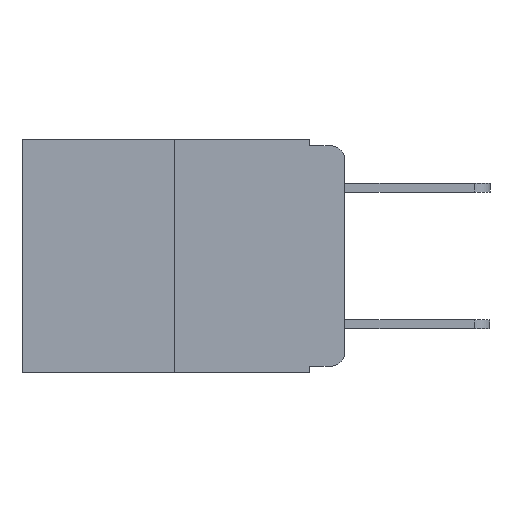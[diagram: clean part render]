
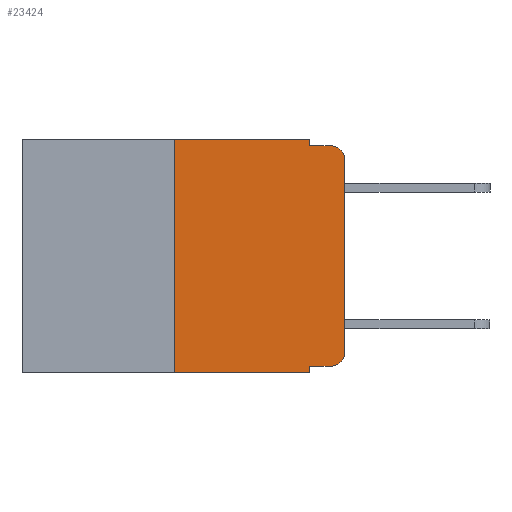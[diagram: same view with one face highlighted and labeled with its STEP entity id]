
A CAD part, left-side view. The second image highlights one B-rep face of the part: STEP entity #23424.
In plain terms, the highlighted planar face has unit normal (-1, 0, 0).
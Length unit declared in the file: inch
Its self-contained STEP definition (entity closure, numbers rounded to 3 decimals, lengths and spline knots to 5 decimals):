
#419 = ORIENTED_EDGE ( 'NONE', *, *, #24900, .T. ) ;
#865 = CARTESIAN_POINT ( 'NONE',  ( 0., 0.473, 0. ) ) ;
#1643 = EDGE_CURVE ( 'NONE', #17742, #3914, #18968, .T. ) ;
#1925 = DIRECTION ( 'NONE',  ( 0., 0., 1. ) ) ;
#2193 = VERTEX_POINT ( 'NONE', #24155 ) ;
#2943 = DIRECTION ( 'NONE',  ( 0., 0., -1. ) ) ;
#3351 = DIRECTION ( 'NONE',  ( 0., 0., 1. ) ) ;
#3469 = ORIENTED_EDGE ( 'NONE', *, *, #14323, .T. ) ;
#3758 = CARTESIAN_POINT ( 'NONE',  ( 0., 0.473, 0. ) ) ;
#3770 = VECTOR ( 'NONE', #12213, 39.37008 ) ;
#3914 = VERTEX_POINT ( 'NONE', #16038 ) ;
#4097 = VERTEX_POINT ( 'NONE', #6999 ) ;
#4697 = VECTOR ( 'NONE', #1925, 39.37008 ) ;
#5209 = CARTESIAN_POINT ( 'NONE',  ( 0., 0.051, -0.343 ) ) ;
#5333 = LINE ( 'NONE', #25013, #20034 ) ;
#5467 = VERTEX_POINT ( 'NONE', #17161 ) ;
#5901 = DIRECTION ( 'NONE',  ( 0., -1., 0. ) ) ;
#6347 = VECTOR ( 'NONE', #17176, 39.37008 ) ;
#6741 = CARTESIAN_POINT ( 'NONE',  ( 0., 0.02, -0.333 ) ) ;
#6977 = CARTESIAN_POINT ( 'NONE',  ( 0., 0., -0.313 ) ) ;
#6999 = CARTESIAN_POINT ( 'NONE',  ( 0., 0.25, -0.343 ) ) ;
#7034 = CARTESIAN_POINT ( 'NONE',  ( 0., 0.02, -0.03 ) ) ;
#7684 = ORIENTED_EDGE ( 'NONE', *, *, #1643, .T. ) ;
#7804 = CARTESIAN_POINT ( 'NONE',  ( 0., 0.051, -0.333 ) ) ;
#8834 = VECTOR ( 'NONE', #3351, 39.37008 ) ;
#8960 = ORIENTED_EDGE ( 'NONE', *, *, #20356, .F. ) ;
#8981 = DIRECTION ( 'NONE',  ( 0., 0., -1. ) ) ;
#9098 = FACE_OUTER_BOUND ( 'NONE', #17158, .T. ) ;
#9564 = CIRCLE ( 'NONE', #15900, 0.02 ) ;
#9618 = EDGE_CURVE ( 'NONE', #5467, #18698, #13600, .T. ) ;
#9799 = DIRECTION ( 'NONE',  ( 0., 0., -1. ) ) ;
#10622 = CARTESIAN_POINT ( 'NONE',  ( 0., 0.02, -0.313 ) ) ;
#10915 = CARTESIAN_POINT ( 'NONE',  ( 0., 0.051, -0.01 ) ) ;
#11240 = CARTESIAN_POINT ( 'NONE',  ( 0., 0.051, 0. ) ) ;
#11308 = EDGE_CURVE ( 'NONE', #18698, #2193, #14424, .T. ) ;
#11548 = CARTESIAN_POINT ( 'NONE',  ( 0., 0.051, -0.333 ) ) ;
#11971 = LINE ( 'NONE', #3758, #6347 ) ;
#12013 = VERTEX_POINT ( 'NONE', #11548 ) ;
#12213 = DIRECTION ( 'NONE',  ( 0., -1., 0. ) ) ;
#12344 = CARTESIAN_POINT ( 'NONE',  ( 0., 0.25, 0. ) ) ;
#12519 = DIRECTION ( 'NONE',  ( 0., 0., -1. ) ) ;
#12824 = VECTOR ( 'NONE', #5901, 39.37008 ) ;
#12828 = DIRECTION ( 'NONE',  ( 0., -1., 0. ) ) ;
#13600 = LINE ( 'NONE', #11240, #18097 ) ;
#14323 = EDGE_CURVE ( 'NONE', #21221, #17742, #23177, .T. ) ;
#14424 = LINE ( 'NONE', #10915, #24014 ) ;
#14495 = DIRECTION ( 'NONE',  ( 1., 0., 0. ) ) ;
#14873 = CARTESIAN_POINT ( 'NONE',  ( 0., 0., 0. ) ) ;
#15462 = ORIENTED_EDGE ( 'NONE', *, *, #24575, .F. ) ;
#15900 = AXIS2_PLACEMENT_3D ( 'NONE', #7034, #20422, #8981 ) ;
#16038 = CARTESIAN_POINT ( 'NONE',  ( 0., 0., -0.03 ) ) ;
#16316 = ORIENTED_EDGE ( 'NONE', *, *, #17960, .F. ) ;
#16337 = PLANE ( 'NONE',  #19644 ) ;
#17153 = VERTEX_POINT ( 'NONE', #5209 ) ;
#17158 = EDGE_LOOP ( 'NONE', ( #7684, #419, #24109, #19073, #16316, #8960, #22121, #15462, #19146, #3469 ) ) ;
#17161 = CARTESIAN_POINT ( 'NONE',  ( 0., 0.051, 0. ) ) ;
#17176 = DIRECTION ( 'NONE',  ( 0., -1., 0. ) ) ;
#17742 = VERTEX_POINT ( 'NONE', #6977 ) ;
#17888 = LINE ( 'NONE', #21809, #3770 ) ;
#17917 = LINE ( 'NONE', #7804, #12824 ) ;
#17960 = EDGE_CURVE ( 'NONE', #23346, #5467, #11971, .T. ) ;
#18097 = VECTOR ( 'NONE', #20932, 39.37008 ) ;
#18698 = VERTEX_POINT ( 'NONE', #23525 ) ;
#18968 = LINE ( 'NONE', #14873, #8834 ) ;
#19040 = EDGE_CURVE ( 'NONE', #12013, #21221, #17917, .T. ) ;
#19073 = ORIENTED_EDGE ( 'NONE', *, *, #9618, .F. ) ;
#19146 = ORIENTED_EDGE ( 'NONE', *, *, #19040, .T. ) ;
#19194 = AXIS2_PLACEMENT_3D ( 'NONE', #10622, #23966, #12519 ) ;
#19644 = AXIS2_PLACEMENT_3D ( 'NONE', #865, #14495, #2943 ) ;
#19676 = LINE ( 'NONE', #24997, #4697 ) ;
#20034 = VECTOR ( 'NONE', #9799, 39.37008 ) ;
#20356 = EDGE_CURVE ( 'NONE', #4097, #23346, #19676, .T. ) ;
#20422 = DIRECTION ( 'NONE',  ( -1., 0., 0. ) ) ;
#20932 = DIRECTION ( 'NONE',  ( 0., 0., -1. ) ) ;
#21221 = VERTEX_POINT ( 'NONE', #6741 ) ;
#21809 = CARTESIAN_POINT ( 'NONE',  ( 0., 0.473, -0.343 ) ) ;
#22121 = ORIENTED_EDGE ( 'NONE', *, *, #24488, .T. ) ;
#23177 = CIRCLE ( 'NONE', #19194, 0.02 ) ;
#23346 = VERTEX_POINT ( 'NONE', #12344 ) ;
#23424 = ADVANCED_FACE ( 'NONE', ( #9098 ), #16337, .F. ) ;
#23525 = CARTESIAN_POINT ( 'NONE',  ( 0., 0.051, -0.01 ) ) ;
#23966 = DIRECTION ( 'NONE',  ( -1., 0., 0. ) ) ;
#24014 = VECTOR ( 'NONE', #12828, 39.37008 ) ;
#24109 = ORIENTED_EDGE ( 'NONE', *, *, #11308, .F. ) ;
#24155 = CARTESIAN_POINT ( 'NONE',  ( 0., 0.02, -0.01 ) ) ;
#24488 = EDGE_CURVE ( 'NONE', #4097, #17153, #17888, .T. ) ;
#24575 = EDGE_CURVE ( 'NONE', #12013, #17153, #5333, .T. ) ;
#24900 = EDGE_CURVE ( 'NONE', #3914, #2193, #9564, .T. ) ;
#24997 = CARTESIAN_POINT ( 'NONE',  ( 0., 0.25, 0. ) ) ;
#25013 = CARTESIAN_POINT ( 'NONE',  ( 0., 0.051, 0. ) ) ;
